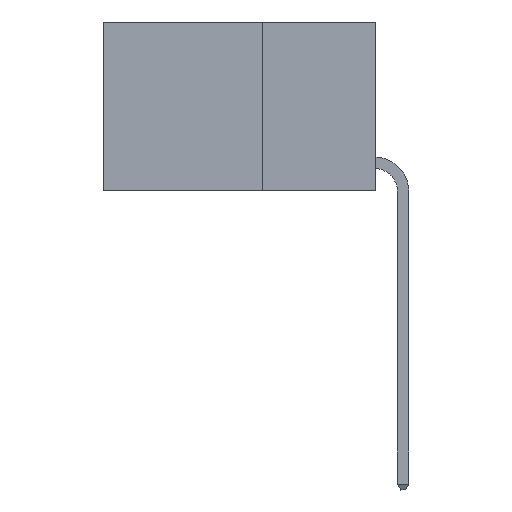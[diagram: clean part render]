
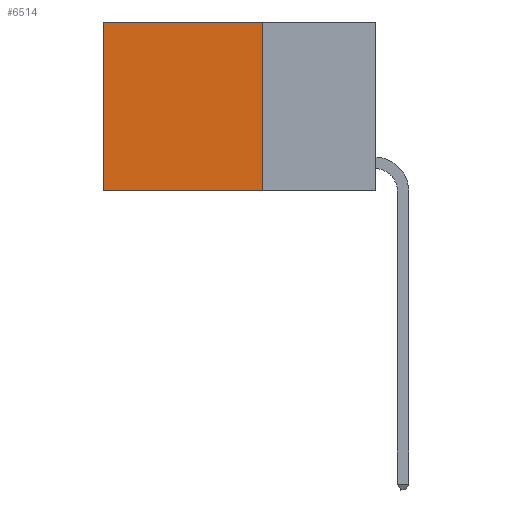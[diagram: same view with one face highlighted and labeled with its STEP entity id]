
A CAD part, left-side view. The second image highlights one B-rep face of the part: STEP entity #6514.
In plain terms, the highlighted planar face has unit normal (-1, 0, 0).
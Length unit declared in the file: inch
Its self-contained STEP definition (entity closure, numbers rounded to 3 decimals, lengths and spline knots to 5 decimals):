
#175 = CARTESIAN_POINT ( 'NONE',  ( 0.2625, 0.6, 0. ) ) ;
#1506 = EDGE_LOOP ( 'NONE', ( #14615, #1562, #10672, #26107 ) ) ;
#1562 = ORIENTED_EDGE ( 'NONE', *, *, #8781, .F. ) ;
#2271 = AXIS2_PLACEMENT_3D ( 'NONE', #23546, #3074, #11699 ) ;
#3074 = DIRECTION ( 'NONE',  ( 1., 0., 0. ) ) ;
#4212 = DIRECTION ( 'NONE',  ( 0., 0., -1. ) ) ;
#4352 = LINE ( 'NONE', #175, #10801 ) ;
#4407 = LINE ( 'NONE', #4995, #9432 ) ;
#4687 = DIRECTION ( 'NONE',  ( 0., 1., 0. ) ) ;
#4995 = CARTESIAN_POINT ( 'NONE',  ( 0.2625, 0.25, 0. ) ) ;
#6514 = ADVANCED_FACE ( 'NONE', ( #23410 ), #27701, .F. ) ;
#6715 = VERTEX_POINT ( 'NONE', #28998 ) ;
#6754 = EDGE_CURVE ( 'NONE', #6715, #22421, #4352, .T. ) ;
#7788 = CARTESIAN_POINT ( 'NONE',  ( 0.2625, 0.25, 0. ) ) ;
#8781 = EDGE_CURVE ( 'NONE', #8871, #22421, #15411, .T. ) ;
#8871 = VERTEX_POINT ( 'NONE', #23414 ) ;
#9150 = VECTOR ( 'NONE', #9630, 39.37008 ) ;
#9279 = CARTESIAN_POINT ( 'NONE',  ( 0.2625, 0.25, -0.37 ) ) ;
#9432 = VECTOR ( 'NONE', #23231, 39.37008 ) ;
#9630 = DIRECTION ( 'NONE',  ( 0., 1., 0. ) ) ;
#9772 = CARTESIAN_POINT ( 'NONE',  ( 0.2625, 0.25, 0. ) ) ;
#10672 = ORIENTED_EDGE ( 'NONE', *, *, #18103, .F. ) ;
#10753 = VERTEX_POINT ( 'NONE', #7788 ) ;
#10801 = VECTOR ( 'NONE', #4212, 39.37008 ) ;
#11699 = DIRECTION ( 'NONE',  ( 0., 0., -1. ) ) ;
#14615 = ORIENTED_EDGE ( 'NONE', *, *, #6754, .T. ) ;
#15411 = LINE ( 'NONE', #9279, #22217 ) ;
#18103 = EDGE_CURVE ( 'NONE', #10753, #8871, #4407, .T. ) ;
#20218 = EDGE_CURVE ( 'NONE', #10753, #6715, #25365, .T. ) ;
#22217 = VECTOR ( 'NONE', #4687, 39.37008 ) ;
#22421 = VERTEX_POINT ( 'NONE', #28784 ) ;
#23231 = DIRECTION ( 'NONE',  ( 0., 0., -1. ) ) ;
#23410 = FACE_OUTER_BOUND ( 'NONE', #1506, .T. ) ;
#23414 = CARTESIAN_POINT ( 'NONE',  ( 0.2625, 0.25, -0.37 ) ) ;
#23546 = CARTESIAN_POINT ( 'NONE',  ( 0.2625, 0.25, 0. ) ) ;
#25365 = LINE ( 'NONE', #9772, #9150 ) ;
#26107 = ORIENTED_EDGE ( 'NONE', *, *, #20218, .T. ) ;
#27701 = PLANE ( 'NONE',  #2271 ) ;
#28784 = CARTESIAN_POINT ( 'NONE',  ( 0.2625, 0.6, -0.37 ) ) ;
#28998 = CARTESIAN_POINT ( 'NONE',  ( 0.2625, 0.6, 0. ) ) ;
